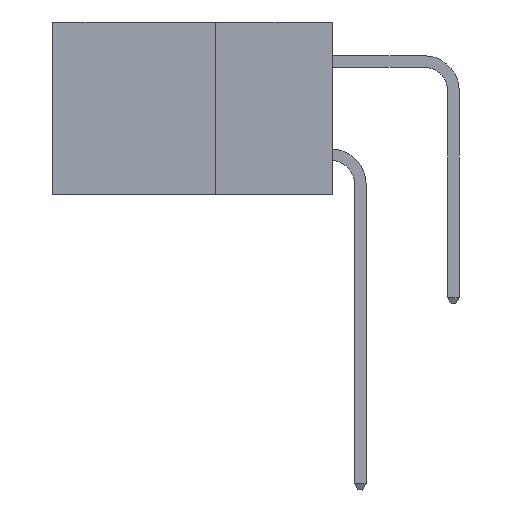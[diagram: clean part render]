
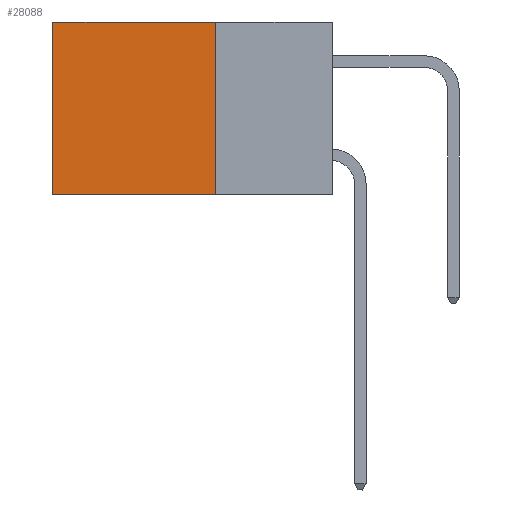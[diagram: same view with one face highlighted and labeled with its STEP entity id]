
A CAD part, left-side view. The second image highlights one B-rep face of the part: STEP entity #28088.
In plain terms, the highlighted planar face has unit normal (-1, 0, 0).
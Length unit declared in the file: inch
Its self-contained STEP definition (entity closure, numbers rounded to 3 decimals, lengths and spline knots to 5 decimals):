
#788 = PLANE ( 'NONE',  #16814 ) ;
#1036 = LINE ( 'NONE', #11017, #15168 ) ;
#1629 = DIRECTION ( 'NONE',  ( 1., 0., 0. ) ) ;
#2300 = LINE ( 'NONE', #18339, #13600 ) ;
#2309 = DIRECTION ( 'NONE',  ( 0., 1., 0. ) ) ;
#2908 = ORIENTED_EDGE ( 'NONE', *, *, #20194, .F. ) ;
#3363 = VERTEX_POINT ( 'NONE', #20881 ) ;
#3599 = DIRECTION ( 'NONE',  ( 0., 0., -1. ) ) ;
#4547 = ORIENTED_EDGE ( 'NONE', *, *, #27342, .F. ) ;
#5060 = FACE_OUTER_BOUND ( 'NONE', #6786, .T. ) ;
#6786 = EDGE_LOOP ( 'NONE', ( #10911, #2908, #4547, #19526 ) ) ;
#7084 = EDGE_CURVE ( 'NONE', #16009, #22439, #1036, .T. ) ;
#8945 = DIRECTION ( 'NONE',  ( 0., 0., -1. ) ) ;
#10911 = ORIENTED_EDGE ( 'NONE', *, *, #7084, .T. ) ;
#11017 = CARTESIAN_POINT ( 'NONE',  ( 0.298, 0.6, 0. ) ) ;
#12022 = VECTOR ( 'NONE', #2309, 39.37008 ) ;
#12366 = CARTESIAN_POINT ( 'NONE',  ( 0.298, 0.25, 0. ) ) ;
#13600 = VECTOR ( 'NONE', #3599, 39.37008 ) ;
#15045 = EDGE_CURVE ( 'NONE', #24685, #16009, #23801, .T. ) ;
#15168 = VECTOR ( 'NONE', #8945, 39.37008 ) ;
#16009 = VERTEX_POINT ( 'NONE', #18692 ) ;
#16814 = AXIS2_PLACEMENT_3D ( 'NONE', #26261, #1629, #28223 ) ;
#17400 = CARTESIAN_POINT ( 'NONE',  ( 0.298, 0.6, -0.37 ) ) ;
#18058 = LINE ( 'NONE', #26733, #12022 ) ;
#18339 = CARTESIAN_POINT ( 'NONE',  ( 0.298, 0.25, 0. ) ) ;
#18692 = CARTESIAN_POINT ( 'NONE',  ( 0.298, 0.6, 0. ) ) ;
#19212 = DIRECTION ( 'NONE',  ( 0., 1., 0. ) ) ;
#19526 = ORIENTED_EDGE ( 'NONE', *, *, #15045, .T. ) ;
#20194 = EDGE_CURVE ( 'NONE', #3363, #22439, #18058, .T. ) ;
#20881 = CARTESIAN_POINT ( 'NONE',  ( 0.298, 0.25, -0.37 ) ) ;
#21669 = VECTOR ( 'NONE', #19212, 39.37008 ) ;
#22439 = VERTEX_POINT ( 'NONE', #17400 ) ;
#23801 = LINE ( 'NONE', #12366, #21669 ) ;
#24685 = VERTEX_POINT ( 'NONE', #25421 ) ;
#25421 = CARTESIAN_POINT ( 'NONE',  ( 0.298, 0.25, 0. ) ) ;
#26261 = CARTESIAN_POINT ( 'NONE',  ( 0.298, 0.25, 0. ) ) ;
#26733 = CARTESIAN_POINT ( 'NONE',  ( 0.298, 0.25, -0.37 ) ) ;
#27342 = EDGE_CURVE ( 'NONE', #24685, #3363, #2300, .T. ) ;
#28088 = ADVANCED_FACE ( 'NONE', ( #5060 ), #788, .F. ) ;
#28223 = DIRECTION ( 'NONE',  ( 0., 0., -1. ) ) ;
